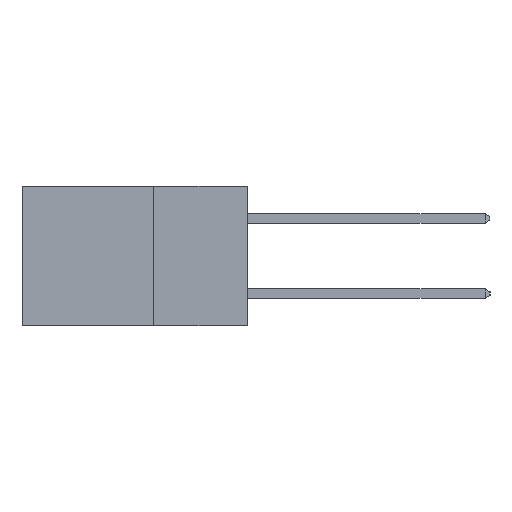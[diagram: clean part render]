
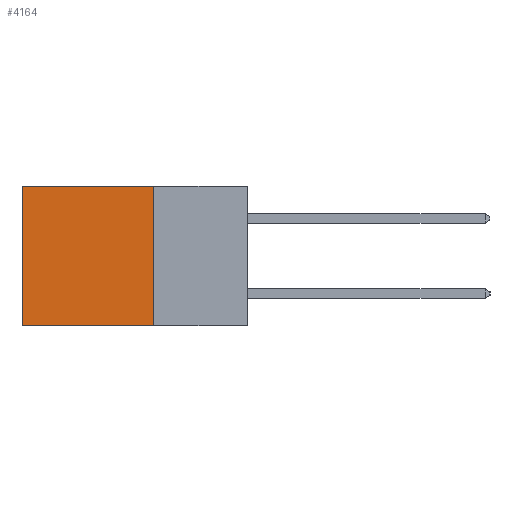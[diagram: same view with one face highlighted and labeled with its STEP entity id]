
A CAD part, left-side view. The second image highlights one B-rep face of the part: STEP entity #4164.
In plain terms, the highlighted planar face has unit normal (-1, 0, 0).
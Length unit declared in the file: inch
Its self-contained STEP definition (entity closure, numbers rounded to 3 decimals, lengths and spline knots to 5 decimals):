
#24 = CARTESIAN_POINT ( 'NONE',  ( 0.2615, 0.6, 0. ) ) ;
#136 = EDGE_CURVE ( 'NONE', #2372, #7210, #3462, .T. ) ;
#166 = VECTOR ( 'NONE', #3236, 39.37008 ) ;
#828 = DIRECTION ( 'NONE',  ( 0., 0., -1. ) ) ;
#842 = CARTESIAN_POINT ( 'NONE',  ( 0.2615, 0.25, -0.37 ) ) ;
#1475 = CARTESIAN_POINT ( 'NONE',  ( 0.2615, 0.25, 0. ) ) ;
#2028 = EDGE_LOOP ( 'NONE', ( #14321, #7066, #6499, #12194 ) ) ;
#2047 = AXIS2_PLACEMENT_3D ( 'NONE', #3808, #3534, #3518 ) ;
#2372 = VERTEX_POINT ( 'NONE', #8711 ) ;
#2796 = EDGE_CURVE ( 'NONE', #6803, #2372, #5730, .T. ) ;
#3236 = DIRECTION ( 'NONE',  ( 0., 1., 0. ) ) ;
#3462 = LINE ( 'NONE', #14023, #166 ) ;
#3518 = DIRECTION ( 'NONE',  ( 0., 0., -1. ) ) ;
#3534 = DIRECTION ( 'NONE',  ( 1., 0., 0. ) ) ;
#3762 = PLANE ( 'NONE',  #2047 ) ;
#3808 = CARTESIAN_POINT ( 'NONE',  ( 0.2615, 0.25, -0.37 ) ) ;
#4164 = ADVANCED_FACE ( 'NONE', ( #5682 ), #3762, .F. ) ;
#4746 = VECTOR ( 'NONE', #9940, 39.37008 ) ;
#5437 = CARTESIAN_POINT ( 'NONE',  ( 0.2615, 0.6, -0.37 ) ) ;
#5456 = DIRECTION ( 'NONE',  ( 0., 0., -1. ) ) ;
#5682 = FACE_OUTER_BOUND ( 'NONE', #2028, .T. ) ;
#5730 = LINE ( 'NONE', #842, #6439 ) ;
#6312 = EDGE_CURVE ( 'NONE', #10697, #7210, #9717, .T. ) ;
#6439 = VECTOR ( 'NONE', #828, 39.37008 ) ;
#6499 = ORIENTED_EDGE ( 'NONE', *, *, #2796, .F. ) ;
#6694 = VECTOR ( 'NONE', #5456, 39.37008 ) ;
#6803 = VERTEX_POINT ( 'NONE', #1475 ) ;
#7066 = ORIENTED_EDGE ( 'NONE', *, *, #136, .F. ) ;
#7210 = VERTEX_POINT ( 'NONE', #8574 ) ;
#7731 = LINE ( 'NONE', #10433, #4746 ) ;
#7926 = EDGE_CURVE ( 'NONE', #6803, #10697, #7731, .T. ) ;
#8574 = CARTESIAN_POINT ( 'NONE',  ( 0.2615, 0.6, -0.37 ) ) ;
#8711 = CARTESIAN_POINT ( 'NONE',  ( 0.2615, 0.25, -0.37 ) ) ;
#9717 = LINE ( 'NONE', #5437, #6694 ) ;
#9940 = DIRECTION ( 'NONE',  ( 0., 1., 0. ) ) ;
#10433 = CARTESIAN_POINT ( 'NONE',  ( 0.2615, 0.25, 0. ) ) ;
#10697 = VERTEX_POINT ( 'NONE', #24 ) ;
#12194 = ORIENTED_EDGE ( 'NONE', *, *, #7926, .T. ) ;
#14023 = CARTESIAN_POINT ( 'NONE',  ( 0.2615, 0.25, -0.37 ) ) ;
#14321 = ORIENTED_EDGE ( 'NONE', *, *, #6312, .T. ) ;
